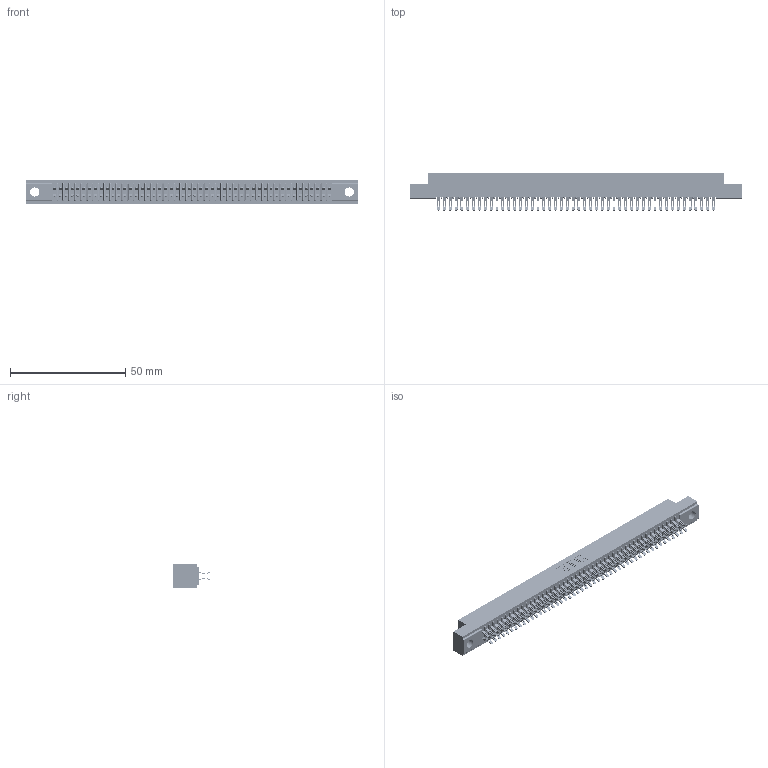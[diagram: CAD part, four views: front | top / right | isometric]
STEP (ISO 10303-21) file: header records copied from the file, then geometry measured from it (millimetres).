
FILE_DESCRIPTION (( 'STEP AP203' ), '1' );
FILE_NAME ('391-096-555-204.STEP', '2018-08-09T18:45:25', ( '' ), ( '' ), 'SwSTEP 2.0', 'SolidWorks 2016', '' );
FILE_SCHEMA (( 'CONFIG_CONTROL_DESIGN' ));
Length unit declared in the file: inch
Products named in the file (3): 391-096-555-204; 341 Part_.156 (3.96) Dia Mounting Holes; 341-292-001_341-292-155
Assembly tree (97 placements, depth 2):
  391-096-555-204
    341 Part_.156 (3.96) Dia Mounting Holes
    341-292-001_341-292-155  x96
Bounding box: 144.15 x 16.31 x 10.16 mm (x, y, z)
Volume: 10665.7 mm3; surface area: 19792.3 mm2
Topology: 97 solids, 97 shells, 7618 faces, 22768 edges, 14822 vertices
Faces by surface type: plane 4114, cylinder 3312, sphere 98, torus 94
Entity records: 58179 total; most frequent: CARTESIAN_POINT 9692, ORIENTED_EDGE 9620, DIRECTION 9384, EDGE_CURVE 4810, LINE 3884, VECTOR 3884, VERTEX_POINT 3042, AXIS2_PLACEMENT_3D 2750
